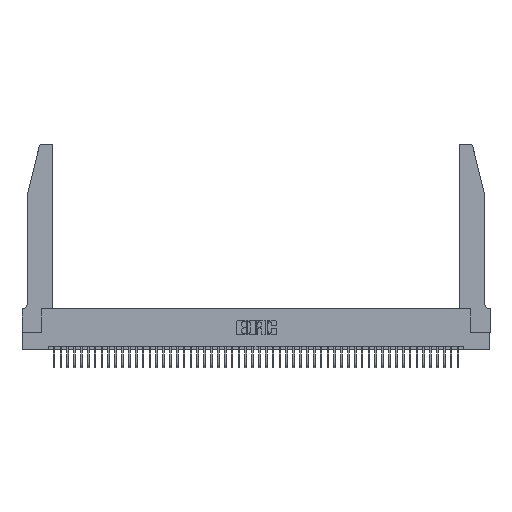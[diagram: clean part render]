
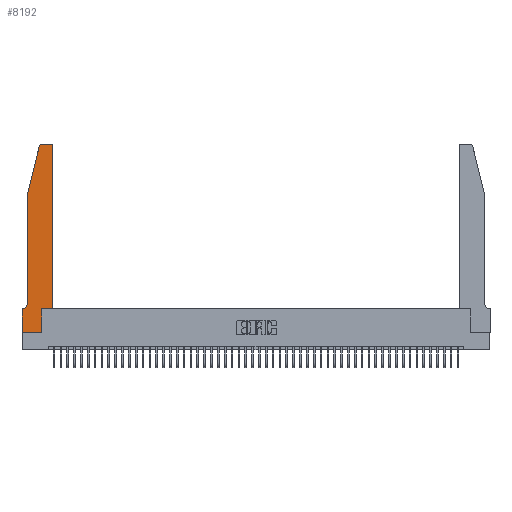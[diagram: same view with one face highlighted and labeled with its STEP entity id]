
A CAD part, top view. The second image highlights one B-rep face of the part: STEP entity #8192.
In plain terms, the highlighted planar face has unit normal (0, 0, 1).
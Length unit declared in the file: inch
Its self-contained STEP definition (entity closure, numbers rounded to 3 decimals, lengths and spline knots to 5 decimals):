
#102 = CARTESIAN_POINT ( 'NONE',  ( 0.4505, 0.35, 0.37 ) ) ;
#741 = VECTOR ( 'NONE', #11561, 39.37008 ) ;
#953 = VECTOR ( 'NONE', #4381, 39.37008 ) ;
#960 = ORIENTED_EDGE ( 'NONE', *, *, #2332, .T. ) ;
#1138 = EDGE_CURVE ( 'NONE', #13665, #41568, #15771, .T. ) ;
#1198 = ORIENTED_EDGE ( 'NONE', *, *, #1138, .T. ) ;
#2108 = LINE ( 'NONE', #22643, #953 ) ;
#2332 = EDGE_CURVE ( 'NONE', #36106, #38662, #23691, .T. ) ;
#2377 = DIRECTION ( 'NONE',  ( 1., 0., 0. ) ) ;
#3809 = DIRECTION ( 'NONE',  ( 0., 1., 0. ) ) ;
#4381 = DIRECTION ( 'NONE',  ( 0., 1., 0. ) ) ;
#4449 = CARTESIAN_POINT ( 'NONE',  ( 0.4505, 0.35, 0.37 ) ) ;
#5191 = DIRECTION ( 'NONE',  ( -0.239, -0.971, 0. ) ) ;
#6324 = VERTEX_POINT ( 'NONE', #9813 ) ;
#8192 = ADVANCED_FACE ( 'NONE', ( #37476 ), #37179, .T. ) ;
#9039 = DIRECTION ( 'NONE',  ( 0., 0., -1. ) ) ;
#9505 = EDGE_CURVE ( 'NONE', #41568, #6324, #26955, .T. ) ;
#9810 = ORIENTED_EDGE ( 'NONE', *, *, #29216, .T. ) ;
#9813 = CARTESIAN_POINT ( 'NONE',  ( 0., 0., 0.37 ) ) ;
#10600 = CARTESIAN_POINT ( 'NONE',  ( 0.2865, 0., 0.37 ) ) ;
#10823 = LINE ( 'NONE', #4449, #13123 ) ;
#11199 = AXIS2_PLACEMENT_3D ( 'NONE', #31045, #9039, #34759 ) ;
#11454 = EDGE_CURVE ( 'NONE', #23778, #36106, #34926, .T. ) ;
#11487 = DIRECTION ( 'NONE',  ( 0., -1., 0. ) ) ;
#11561 = DIRECTION ( 'NONE',  ( -1., 0., 0. ) ) ;
#12984 = LINE ( 'NONE', #46929, #21598 ) ;
#13123 = VECTOR ( 'NONE', #30124, 39.37008 ) ;
#13213 = ORIENTED_EDGE ( 'NONE', *, *, #35900, .T. ) ;
#13665 = VERTEX_POINT ( 'NONE', #22866 ) ;
#14002 = CARTESIAN_POINT ( 'NONE',  ( 0.284, 2.72, 0.37 ) ) ;
#14364 = CARTESIAN_POINT ( 'NONE',  ( 0.4505, 2.72, 0.37 ) ) ;
#14642 = CARTESIAN_POINT ( 'NONE',  ( 0.4505, 0.35, 0.37 ) ) ;
#15125 = DIRECTION ( 'NONE',  ( 0., 0., 1. ) ) ;
#15771 = LINE ( 'NONE', #46653, #43905 ) ;
#16698 = ORIENTED_EDGE ( 'NONE', *, *, #28402, .T. ) ;
#17510 = AXIS2_PLACEMENT_3D ( 'NONE', #14002, #39752, #17689 ) ;
#17672 = DIRECTION ( 'NONE',  ( 1., 0., 0. ) ) ;
#17689 = DIRECTION ( 'NONE',  ( 1., 0., 0. ) ) ;
#18382 = CARTESIAN_POINT ( 'NONE',  ( 0.0755, 0.42, 0.37 ) ) ;
#18607 = EDGE_LOOP ( 'NONE', ( #960, #13213, #9810, #43160, #35212, #1198, #20574, #19892, #42977, #16698, #43904, #27021 ) ) ;
#18942 = CARTESIAN_POINT ( 'NONE',  ( 0.4205, 2.75, 0.37 ) ) ;
#19030 = EDGE_CURVE ( 'NONE', #21308, #13665, #43430, .T. ) ;
#19892 = ORIENTED_EDGE ( 'NONE', *, *, #30500, .T. ) ;
#20574 = ORIENTED_EDGE ( 'NONE', *, *, #9505, .T. ) ;
#20762 = LINE ( 'NONE', #22908, #39169 ) ;
#21308 = VERTEX_POINT ( 'NONE', #18382 ) ;
#21598 = VECTOR ( 'NONE', #17672, 39.37008 ) ;
#22643 = CARTESIAN_POINT ( 'NONE',  ( 0.2865, 0.35, 0.37 ) ) ;
#22866 = CARTESIAN_POINT ( 'NONE',  ( 0.0055, 0.35, 0.37 ) ) ;
#22908 = CARTESIAN_POINT ( 'NONE',  ( 0.0755, 2., 0.37 ) ) ;
#23448 = CARTESIAN_POINT ( 'NONE',  ( 0.0755, 2., 0.37 ) ) ;
#23691 = LINE ( 'NONE', #26196, #741 ) ;
#23778 = VERTEX_POINT ( 'NONE', #14364 ) ;
#24351 = DIRECTION ( 'NONE',  ( 0., 0., 1. ) ) ;
#24620 = LINE ( 'NONE', #23448, #33277 ) ;
#25744 = CIRCLE ( 'NONE', #17510, 0.03 ) ;
#26196 = CARTESIAN_POINT ( 'NONE',  ( 0.2605, 2.75, 0.37 ) ) ;
#26632 = DIRECTION ( 'NONE',  ( 0., -1., 0. ) ) ;
#26955 = LINE ( 'NONE', #33696, #37893 ) ;
#27021 = ORIENTED_EDGE ( 'NONE', *, *, #11454, .T. ) ;
#27674 = CARTESIAN_POINT ( 'NONE',  ( 0.25487, 2.72718, 0.37 ) ) ;
#28402 = EDGE_CURVE ( 'NONE', #31999, #34158, #10823, .T. ) ;
#28408 = CARTESIAN_POINT ( 'NONE',  ( 0.2865, 0.35, 0.37 ) ) ;
#29216 = EDGE_CURVE ( 'NONE', #46748, #38268, #24620, .T. ) ;
#30006 = EDGE_CURVE ( 'NONE', #34158, #23778, #36052, .T. ) ;
#30124 = DIRECTION ( 'NONE',  ( 1., 0., 0. ) ) ;
#30500 = EDGE_CURVE ( 'NONE', #6324, #46922, #12984, .T. ) ;
#31045 = CARTESIAN_POINT ( 'NONE',  ( 0.0055, 0.42, 0.37 ) ) ;
#31922 = DIRECTION ( 'NONE',  ( -1., 0., 0. ) ) ;
#31999 = VERTEX_POINT ( 'NONE', #28408 ) ;
#32556 = CARTESIAN_POINT ( 'NONE',  ( 0., 0.35, 0.37 ) ) ;
#32610 = VECTOR ( 'NONE', #3809, 39.37008 ) ;
#33277 = VECTOR ( 'NONE', #5191, 39.37008 ) ;
#33696 = CARTESIAN_POINT ( 'NONE',  ( 0., 0., 0.37 ) ) ;
#34158 = VERTEX_POINT ( 'NONE', #14642 ) ;
#34759 = DIRECTION ( 'NONE',  ( -1., 0., 0. ) ) ;
#34926 = CIRCLE ( 'NONE', #37206, 0.03 ) ;
#35212 = ORIENTED_EDGE ( 'NONE', *, *, #19030, .T. ) ;
#35900 = EDGE_CURVE ( 'NONE', #38662, #46748, #25744, .T. ) ;
#36052 = LINE ( 'NONE', #102, #32610 ) ;
#36106 = VERTEX_POINT ( 'NONE', #18942 ) ;
#37162 = EDGE_CURVE ( 'NONE', #46922, #31999, #2108, .T. ) ;
#37179 = PLANE ( 'NONE',  #46333 ) ;
#37206 = AXIS2_PLACEMENT_3D ( 'NONE', #46351, #24351, #2377 ) ;
#37476 = FACE_OUTER_BOUND ( 'NONE', #18607, .T. ) ;
#37893 = VECTOR ( 'NONE', #11487, 39.37008 ) ;
#38268 = VERTEX_POINT ( 'NONE', #40547 ) ;
#38662 = VERTEX_POINT ( 'NONE', #39102 ) ;
#39102 = CARTESIAN_POINT ( 'NONE',  ( 0.284, 2.75, 0.37 ) ) ;
#39169 = VECTOR ( 'NONE', #26632, 39.37008 ) ;
#39752 = DIRECTION ( 'NONE',  ( 0., 0., 1. ) ) ;
#40547 = CARTESIAN_POINT ( 'NONE',  ( 0.0755, 2., 0.37 ) ) ;
#40840 = DIRECTION ( 'NONE',  ( 1., 0., 0. ) ) ;
#41568 = VERTEX_POINT ( 'NONE', #32556 ) ;
#42977 = ORIENTED_EDGE ( 'NONE', *, *, #37162, .T. ) ;
#43160 = ORIENTED_EDGE ( 'NONE', *, *, #45041, .T. ) ;
#43430 = CIRCLE ( 'NONE', #11199, 0.07 ) ;
#43904 = ORIENTED_EDGE ( 'NONE', *, *, #30006, .T. ) ;
#43905 = VECTOR ( 'NONE', #31922, 39.37008 ) ;
#44347 = CARTESIAN_POINT ( 'NONE',  ( 0., 0.35, 0.37 ) ) ;
#45041 = EDGE_CURVE ( 'NONE', #38268, #21308, #20762, .T. ) ;
#46333 = AXIS2_PLACEMENT_3D ( 'NONE', #44347, #15125, #40840 ) ;
#46351 = CARTESIAN_POINT ( 'NONE',  ( 0.4205, 2.72, 0.37 ) ) ;
#46653 = CARTESIAN_POINT ( 'NONE',  ( 0.0755, 0.35, 0.37 ) ) ;
#46748 = VERTEX_POINT ( 'NONE', #27674 ) ;
#46922 = VERTEX_POINT ( 'NONE', #10600 ) ;
#46929 = CARTESIAN_POINT ( 'NONE',  ( 0., 0., 0.37 ) ) ;
